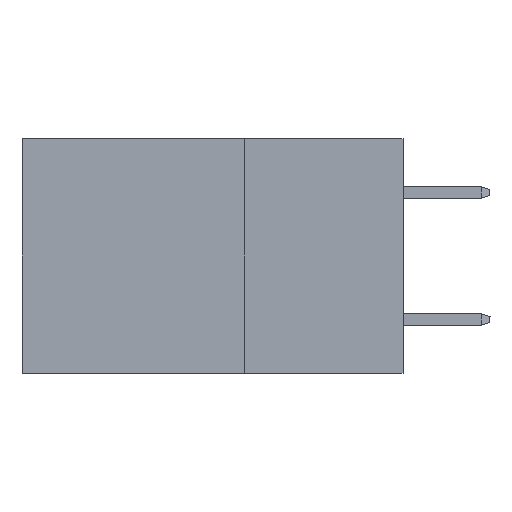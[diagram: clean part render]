
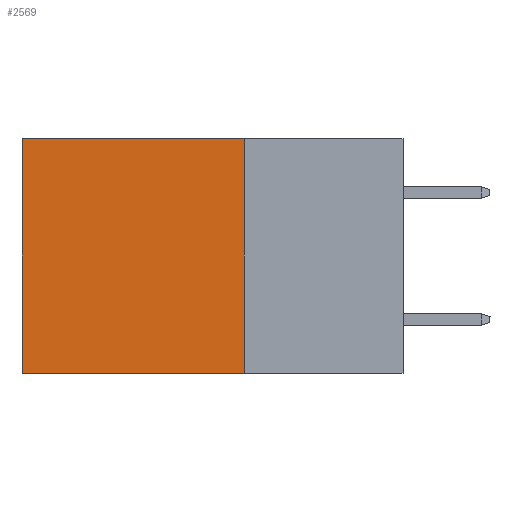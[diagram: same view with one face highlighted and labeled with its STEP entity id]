
A CAD part, left-side view. The second image highlights one B-rep face of the part: STEP entity #2569.
In plain terms, the highlighted planar face has unit normal (-1, 0, 0).
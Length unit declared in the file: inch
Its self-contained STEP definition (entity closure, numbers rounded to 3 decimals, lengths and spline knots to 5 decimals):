
#119 = ORIENTED_EDGE ( 'NONE', *, *, #17317, .T. ) ;
#258 = EDGE_CURVE ( 'NONE', #9509, #17311, #698, .T. ) ;
#445 = CARTESIAN_POINT ( 'NONE',  ( 0.2875, 0.6, 0. ) ) ;
#698 = LINE ( 'NONE', #1761, #1245 ) ;
#1245 = VECTOR ( 'NONE', #6526, 39.37008 ) ;
#1761 = CARTESIAN_POINT ( 'NONE',  ( 0.2875, 0.25, 0. ) ) ;
#1929 = AXIS2_PLACEMENT_3D ( 'NONE', #2573, #11706, #18994 ) ;
#1950 = LINE ( 'NONE', #9260, #15409 ) ;
#2096 = CARTESIAN_POINT ( 'NONE',  ( 0.2875, 0.25, -0.37 ) ) ;
#2569 = ADVANCED_FACE ( 'NONE', ( #6880 ), #11613, .F. ) ;
#2573 = CARTESIAN_POINT ( 'NONE',  ( 0.2875, 0.25, 0. ) ) ;
#4219 = EDGE_CURVE ( 'NONE', #11123, #6065, #15459, .T. ) ;
#4616 = DIRECTION ( 'NONE',  ( 0., 0., -1. ) ) ;
#6065 = VERTEX_POINT ( 'NONE', #10860 ) ;
#6149 = VECTOR ( 'NONE', #4616, 39.37008 ) ;
#6526 = DIRECTION ( 'NONE',  ( 0., 1., 0. ) ) ;
#6880 = FACE_OUTER_BOUND ( 'NONE', #17668, .T. ) ;
#7451 = ORIENTED_EDGE ( 'NONE', *, *, #4219, .F. ) ;
#9089 = ORIENTED_EDGE ( 'NONE', *, *, #258, .T. ) ;
#9260 = CARTESIAN_POINT ( 'NONE',  ( 0.2875, 0.25, 0. ) ) ;
#9473 = CARTESIAN_POINT ( 'NONE',  ( 0.2875, 0.25, -0.37 ) ) ;
#9509 = VERTEX_POINT ( 'NONE', #17970 ) ;
#9753 = VECTOR ( 'NONE', #11054, 39.37008 ) ;
#10860 = CARTESIAN_POINT ( 'NONE',  ( 0.2875, 0.6, -0.37 ) ) ;
#11054 = DIRECTION ( 'NONE',  ( 0., 1., 0. ) ) ;
#11123 = VERTEX_POINT ( 'NONE', #9473 ) ;
#11453 = ORIENTED_EDGE ( 'NONE', *, *, #12677, .F. ) ;
#11613 = PLANE ( 'NONE',  #1929 ) ;
#11706 = DIRECTION ( 'NONE',  ( 1., 0., 0. ) ) ;
#12677 = EDGE_CURVE ( 'NONE', #9509, #11123, #1950, .T. ) ;
#13554 = DIRECTION ( 'NONE',  ( 0., 0., -1. ) ) ;
#15332 = LINE ( 'NONE', #15431, #6149 ) ;
#15409 = VECTOR ( 'NONE', #13554, 39.37008 ) ;
#15431 = CARTESIAN_POINT ( 'NONE',  ( 0.2875, 0.6, 0. ) ) ;
#15459 = LINE ( 'NONE', #2096, #9753 ) ;
#17311 = VERTEX_POINT ( 'NONE', #445 ) ;
#17317 = EDGE_CURVE ( 'NONE', #17311, #6065, #15332, .T. ) ;
#17668 = EDGE_LOOP ( 'NONE', ( #119, #7451, #11453, #9089 ) ) ;
#17970 = CARTESIAN_POINT ( 'NONE',  ( 0.2875, 0.25, 0. ) ) ;
#18994 = DIRECTION ( 'NONE',  ( 0., 0., -1. ) ) ;
